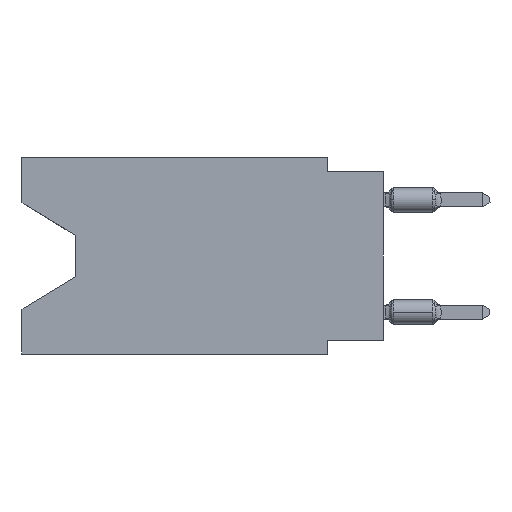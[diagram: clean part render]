
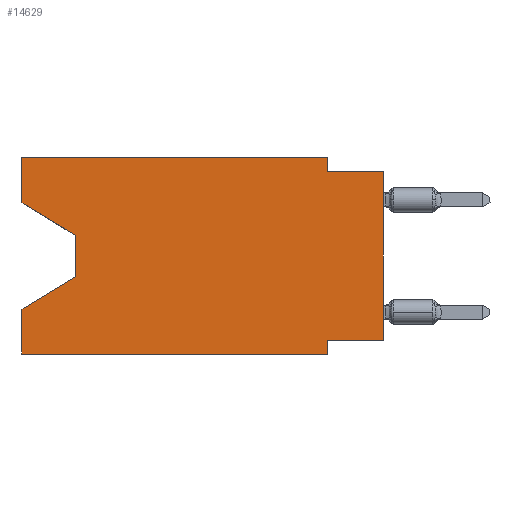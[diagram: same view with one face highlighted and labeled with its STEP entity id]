
A CAD part, left-side view. The second image highlights one B-rep face of the part: STEP entity #14629.
In plain terms, the highlighted planar face has unit normal (-1, 0, 0).
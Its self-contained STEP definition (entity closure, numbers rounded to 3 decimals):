
#65 = LINE ( 'NONE', #4611, #5147 ) ;
#198 = EDGE_CURVE ( 'NONE', #15078, #3292, #4113, .T. ) ;
#334 = EDGE_CURVE ( 'NONE', #12769, #15107, #1920, .T. ) ;
#373 = VECTOR ( 'NONE', #9561, 1000. ) ;
#462 = VERTEX_POINT ( 'NONE', #14434 ) ;
#674 = DIRECTION ( 'NONE',  ( 0., 0., -1. ) ) ;
#1265 = CARTESIAN_POINT ( 'NONE',  ( 0., 16.383, -2.038 ) ) ;
#1359 = VECTOR ( 'NONE', #5538, 1000. ) ;
#1463 = LINE ( 'NONE', #8696, #3651 ) ;
#1920 = LINE ( 'NONE', #6642, #11263 ) ;
#2082 = ORIENTED_EDGE ( 'NONE', *, *, #4596, .T. ) ;
#2247 = VECTOR ( 'NONE', #12431, 1000. ) ;
#2282 = VERTEX_POINT ( 'NONE', #10009 ) ;
#2294 = ORIENTED_EDGE ( 'NONE', *, *, #4720, .F. ) ;
#2993 = ORIENTED_EDGE ( 'NONE', *, *, #3668, .F. ) ;
#3163 = VECTOR ( 'NONE', #11307, 1000. ) ;
#3210 = ORIENTED_EDGE ( 'NONE', *, *, #4456, .F. ) ;
#3292 = VERTEX_POINT ( 'NONE', #5948 ) ;
#3486 = CARTESIAN_POINT ( 'NONE',  ( 0., 2.54, -8.89 ) ) ;
#3533 = ORIENTED_EDGE ( 'NONE', *, *, #12356, .F. ) ;
#3557 = LINE ( 'NONE', #3486, #373 ) ;
#3645 = DIRECTION ( 'NONE',  ( 0., 0., 1. ) ) ;
#3651 = VECTOR ( 'NONE', #13354, 1000. ) ;
#3668 = EDGE_CURVE ( 'NONE', #10361, #4425, #3557, .T. ) ;
#4012 = ORIENTED_EDGE ( 'NONE', *, *, #4146, .T. ) ;
#4069 = DIRECTION ( 'NONE',  ( 1., 0., 0. ) ) ;
#4113 = LINE ( 'NONE', #7755, #3163 ) ;
#4142 = PLANE ( 'NONE',  #5524 ) ;
#4146 = EDGE_CURVE ( 'NONE', #11533, #11192, #8340, .T. ) ;
#4283 = CARTESIAN_POINT ( 'NONE',  ( 0., 16.383, -8.89 ) ) ;
#4425 = VERTEX_POINT ( 'NONE', #5718 ) ;
#4456 = EDGE_CURVE ( 'NONE', #2282, #12769, #65, .T. ) ;
#4521 = VERTEX_POINT ( 'NONE', #10692 ) ;
#4596 = EDGE_CURVE ( 'NONE', #11192, #4521, #9731, .T. ) ;
#4611 = CARTESIAN_POINT ( 'NONE',  ( 0., 16.383, 0. ) ) ;
#4720 = EDGE_CURVE ( 'NONE', #11533, #2282, #1463, .T. ) ;
#4913 = ORIENTED_EDGE ( 'NONE', *, *, #15171, .T. ) ;
#4970 = CARTESIAN_POINT ( 'NONE',  ( 0., 16.383, 0. ) ) ;
#5147 = VECTOR ( 'NONE', #12031, 1000. ) ;
#5390 = ORIENTED_EDGE ( 'NONE', *, *, #5534, .T. ) ;
#5403 = FACE_OUTER_BOUND ( 'NONE', #11520, .T. ) ;
#5524 = AXIS2_PLACEMENT_3D ( 'NONE', #12430, #4069, #7782 ) ;
#5534 = EDGE_CURVE ( 'NONE', #4521, #7897, #12813, .T. ) ;
#5538 = DIRECTION ( 'NONE',  ( 0., -1., 0. ) ) ;
#5718 = CARTESIAN_POINT ( 'NONE',  ( 0., 2.54, -8.89 ) ) ;
#5948 = CARTESIAN_POINT ( 'NONE',  ( 0., 0., -0.635 ) ) ;
#6513 = CARTESIAN_POINT ( 'NONE',  ( 0., 2.54, -8.255 ) ) ;
#6607 = ORIENTED_EDGE ( 'NONE', *, *, #8575, .F. ) ;
#6642 = CARTESIAN_POINT ( 'NONE',  ( 0., 2.54, 0. ) ) ;
#6820 = DIRECTION ( 'NONE',  ( 0., 0.855, -0.519 ) ) ;
#7204 = LINE ( 'NONE', #4970, #9183 ) ;
#7575 = LINE ( 'NONE', #7739, #10128 ) ;
#7719 = CARTESIAN_POINT ( 'NONE',  ( 0., 16.383, -6.852 ) ) ;
#7739 = CARTESIAN_POINT ( 'NONE',  ( 0., 0., -8.255 ) ) ;
#7755 = CARTESIAN_POINT ( 'NONE',  ( 0., 0., 0. ) ) ;
#7782 = DIRECTION ( 'NONE',  ( 0., 0., -1. ) ) ;
#7897 = VERTEX_POINT ( 'NONE', #7719 ) ;
#8290 = EDGE_CURVE ( 'NONE', #15107, #3292, #8642, .T. ) ;
#8340 = LINE ( 'NONE', #1265, #14463 ) ;
#8575 = EDGE_CURVE ( 'NONE', #462, #7897, #7204, .T. ) ;
#8642 = LINE ( 'NONE', #12197, #2247 ) ;
#8696 = CARTESIAN_POINT ( 'NONE',  ( 0., 16.383, 0. ) ) ;
#8890 = CARTESIAN_POINT ( 'NONE',  ( 0., 16.383, -2.038 ) ) ;
#8909 = DIRECTION ( 'NONE',  ( 0., 1., 0. ) ) ;
#9068 = CARTESIAN_POINT ( 'NONE',  ( 0., 13.97, -3.505 ) ) ;
#9183 = VECTOR ( 'NONE', #3645, 1000. ) ;
#9561 = DIRECTION ( 'NONE',  ( 0., 0., -1. ) ) ;
#9731 = LINE ( 'NONE', #15484, #10204 ) ;
#10009 = CARTESIAN_POINT ( 'NONE',  ( 0., 16.383, 0. ) ) ;
#10128 = VECTOR ( 'NONE', #8909, 1000. ) ;
#10204 = VECTOR ( 'NONE', #14387, 1000. ) ;
#10279 = CARTESIAN_POINT ( 'NONE',  ( 0., 2.54, -0.635 ) ) ;
#10361 = VERTEX_POINT ( 'NONE', #6513 ) ;
#10692 = CARTESIAN_POINT ( 'NONE',  ( 0., 13.97, -5.385 ) ) ;
#11130 = ORIENTED_EDGE ( 'NONE', *, *, #198, .T. ) ;
#11192 = VERTEX_POINT ( 'NONE', #9068 ) ;
#11263 = VECTOR ( 'NONE', #674, 1000. ) ;
#11307 = DIRECTION ( 'NONE',  ( 0., 0., 1. ) ) ;
#11520 = EDGE_LOOP ( 'NONE', ( #4012, #2082, #5390, #6607, #4913, #2993, #3533, #11130, #14150, #13055, #3210, #2294 ) ) ;
#11533 = VERTEX_POINT ( 'NONE', #8890 ) ;
#11575 = CARTESIAN_POINT ( 'NONE',  ( 0., 2.54, 0. ) ) ;
#12031 = DIRECTION ( 'NONE',  ( 0., -1., 0. ) ) ;
#12197 = CARTESIAN_POINT ( 'NONE',  ( 0., 0., -0.635 ) ) ;
#12356 = EDGE_CURVE ( 'NONE', #15078, #10361, #7575, .T. ) ;
#12430 = CARTESIAN_POINT ( 'NONE',  ( 0., 16.383, 0. ) ) ;
#12431 = DIRECTION ( 'NONE',  ( 0., -1., 0. ) ) ;
#12769 = VERTEX_POINT ( 'NONE', #11575 ) ;
#12813 = LINE ( 'NONE', #14235, #15296 ) ;
#13055 = ORIENTED_EDGE ( 'NONE', *, *, #334, .F. ) ;
#13074 = DIRECTION ( 'NONE',  ( 0., -0.855, -0.519 ) ) ;
#13354 = DIRECTION ( 'NONE',  ( 0., 0., 1. ) ) ;
#13902 = LINE ( 'NONE', #4283, #1359 ) ;
#14150 = ORIENTED_EDGE ( 'NONE', *, *, #8290, .F. ) ;
#14235 = CARTESIAN_POINT ( 'NONE',  ( 0., 13.97, -5.385 ) ) ;
#14387 = DIRECTION ( 'NONE',  ( 0., 0., -1. ) ) ;
#14434 = CARTESIAN_POINT ( 'NONE',  ( 0., 16.383, -8.89 ) ) ;
#14463 = VECTOR ( 'NONE', #13074, 1000. ) ;
#14629 = ADVANCED_FACE ( 'NONE', ( #5403 ), #4142, .F. ) ;
#15078 = VERTEX_POINT ( 'NONE', #15316 ) ;
#15107 = VERTEX_POINT ( 'NONE', #10279 ) ;
#15171 = EDGE_CURVE ( 'NONE', #462, #4425, #13902, .T. ) ;
#15296 = VECTOR ( 'NONE', #6820, 1000. ) ;
#15316 = CARTESIAN_POINT ( 'NONE',  ( 0., 0., -8.255 ) ) ;
#15484 = CARTESIAN_POINT ( 'NONE',  ( 0., 13.97, -3.505 ) ) ;
